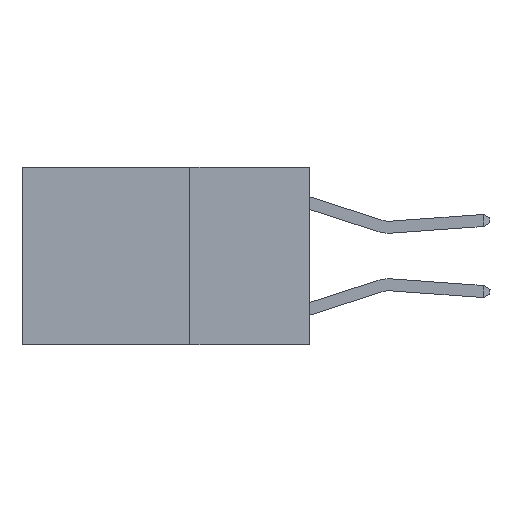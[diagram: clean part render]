
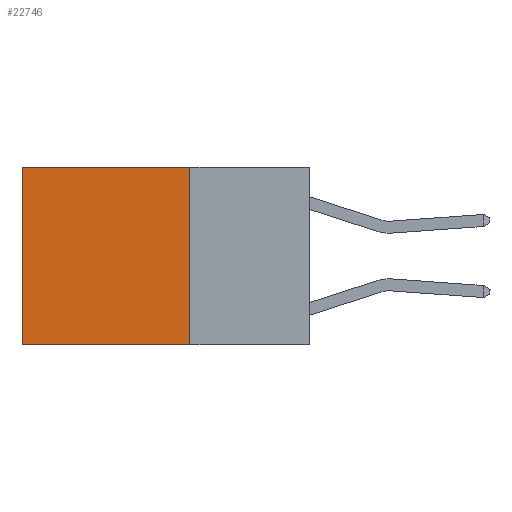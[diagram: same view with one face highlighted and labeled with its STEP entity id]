
A CAD part, left-side view. The second image highlights one B-rep face of the part: STEP entity #22746.
In plain terms, the highlighted planar face has unit normal (-1, 0, 0).
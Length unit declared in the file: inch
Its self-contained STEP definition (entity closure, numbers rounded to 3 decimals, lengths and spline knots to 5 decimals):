
#304 = DIRECTION ( 'NONE',  ( 0., 1., 0. ) ) ;
#1771 = ORIENTED_EDGE ( 'NONE', *, *, #16657, .T. ) ;
#2144 = CARTESIAN_POINT ( 'NONE',  ( 0.2625, 0.25, 0. ) ) ;
#2495 = VECTOR ( 'NONE', #14230, 39.37008 ) ;
#2658 = DIRECTION ( 'NONE',  ( 0., 1., 0. ) ) ;
#3108 = LINE ( 'NONE', #4746, #2495 ) ;
#3685 = PLANE ( 'NONE',  #6897 ) ;
#4400 = VERTEX_POINT ( 'NONE', #19958 ) ;
#4746 = CARTESIAN_POINT ( 'NONE',  ( 0.2625, 0.25, 0. ) ) ;
#5232 = CARTESIAN_POINT ( 'NONE',  ( 0.2625, 0.6, 0. ) ) ;
#5625 = DIRECTION ( 'NONE',  ( 0., 0., -1. ) ) ;
#5727 = VECTOR ( 'NONE', #20941, 39.37008 ) ;
#5781 = EDGE_CURVE ( 'NONE', #4400, #22483, #3108, .T. ) ;
#6390 = VERTEX_POINT ( 'NONE', #11915 ) ;
#6897 = AXIS2_PLACEMENT_3D ( 'NONE', #9406, #17025, #5625 ) ;
#7177 = EDGE_CURVE ( 'NONE', #22483, #6390, #22013, .T. ) ;
#7656 = EDGE_CURVE ( 'NONE', #15706, #6390, #20873, .T. ) ;
#8995 = EDGE_LOOP ( 'NONE', ( #12163, #15964, #10252, #1771 ) ) ;
#9406 = CARTESIAN_POINT ( 'NONE',  ( 0.2625, 0.25, 0. ) ) ;
#9559 = VECTOR ( 'NONE', #304, 39.37008 ) ;
#10252 = ORIENTED_EDGE ( 'NONE', *, *, #5781, .F. ) ;
#11915 = CARTESIAN_POINT ( 'NONE',  ( 0.2625, 0.6, -0.37 ) ) ;
#12163 = ORIENTED_EDGE ( 'NONE', *, *, #7656, .T. ) ;
#14230 = DIRECTION ( 'NONE',  ( 0., 0., -1. ) ) ;
#14274 = CARTESIAN_POINT ( 'NONE',  ( 0.2625, 0.25, -0.37 ) ) ;
#15178 = LINE ( 'NONE', #2144, #9559 ) ;
#15248 = CARTESIAN_POINT ( 'NONE',  ( 0.2625, 0.6, 0. ) ) ;
#15706 = VERTEX_POINT ( 'NONE', #5232 ) ;
#15855 = VECTOR ( 'NONE', #2658, 39.37008 ) ;
#15964 = ORIENTED_EDGE ( 'NONE', *, *, #7177, .F. ) ;
#16005 = CARTESIAN_POINT ( 'NONE',  ( 0.2625, 0.25, -0.37 ) ) ;
#16657 = EDGE_CURVE ( 'NONE', #4400, #15706, #15178, .T. ) ;
#17025 = DIRECTION ( 'NONE',  ( 1., 0., 0. ) ) ;
#19958 = CARTESIAN_POINT ( 'NONE',  ( 0.2625, 0.25, 0. ) ) ;
#20873 = LINE ( 'NONE', #15248, #5727 ) ;
#20941 = DIRECTION ( 'NONE',  ( 0., 0., -1. ) ) ;
#21754 = FACE_OUTER_BOUND ( 'NONE', #8995, .T. ) ;
#22013 = LINE ( 'NONE', #16005, #15855 ) ;
#22483 = VERTEX_POINT ( 'NONE', #14274 ) ;
#22746 = ADVANCED_FACE ( 'NONE', ( #21754 ), #3685, .F. ) ;
